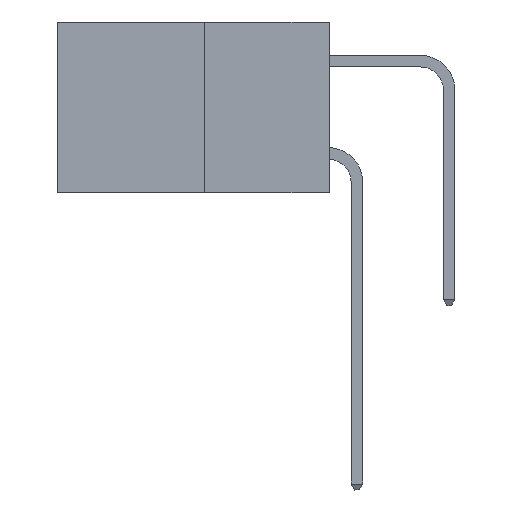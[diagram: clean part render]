
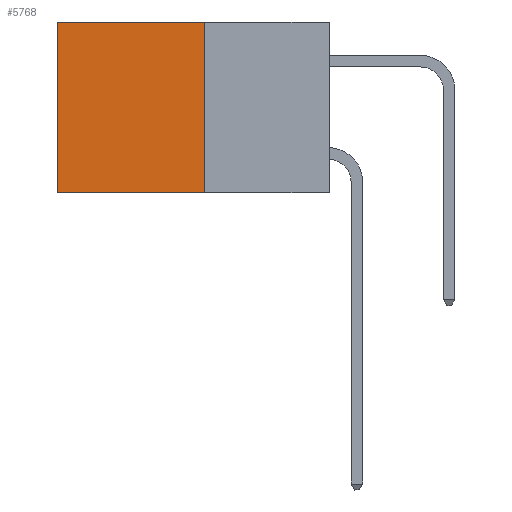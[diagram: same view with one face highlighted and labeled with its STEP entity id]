
A CAD part, left-side view. The second image highlights one B-rep face of the part: STEP entity #5768.
In plain terms, the highlighted planar face has unit normal (-1, 0, 0).
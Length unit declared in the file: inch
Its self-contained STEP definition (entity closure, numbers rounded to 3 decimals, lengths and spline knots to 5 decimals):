
#356 = CARTESIAN_POINT ( 'NONE',  ( 0.277, 0.27, -0.37 ) ) ;
#389 = VERTEX_POINT ( 'NONE', #7781 ) ;
#3956 = CARTESIAN_POINT ( 'NONE',  ( 0.277, 0.27, -0.37 ) ) ;
#4739 = VECTOR ( 'NONE', #16791, 39.37008 ) ;
#4917 = ORIENTED_EDGE ( 'NONE', *, *, #9083, .F. ) ;
#5041 = LINE ( 'NONE', #356, #25148 ) ;
#5121 = PLANE ( 'NONE',  #22793 ) ;
#5768 = ADVANCED_FACE ( 'NONE', ( #12436 ), #5121, .F. ) ;
#5846 = CARTESIAN_POINT ( 'NONE',  ( 0.277, 0.27, 0. ) ) ;
#6281 = DIRECTION ( 'NONE',  ( 0., 0., -1. ) ) ;
#6691 = DIRECTION ( 'NONE',  ( 0., 0., -1. ) ) ;
#7781 = CARTESIAN_POINT ( 'NONE',  ( 0.277, 0.59, -0.37 ) ) ;
#8143 = CARTESIAN_POINT ( 'NONE',  ( 0.277, 0.59, 0. ) ) ;
#9062 = DIRECTION ( 'NONE',  ( 0., 0., -1. ) ) ;
#9083 = EDGE_CURVE ( 'NONE', #11509, #16368, #5041, .T. ) ;
#9275 = EDGE_LOOP ( 'NONE', ( #20755, #25209, #4917, #24793 ) ) ;
#11509 = VERTEX_POINT ( 'NONE', #5846 ) ;
#12280 = DIRECTION ( 'NONE',  ( 0., 1., 0. ) ) ;
#12358 = VECTOR ( 'NONE', #6691, 39.37008 ) ;
#12436 = FACE_OUTER_BOUND ( 'NONE', #9275, .T. ) ;
#14859 = CARTESIAN_POINT ( 'NONE',  ( 0.277, 0.27, -0.37 ) ) ;
#15082 = VERTEX_POINT ( 'NONE', #8143 ) ;
#15148 = LINE ( 'NONE', #14859, #4739 ) ;
#16368 = VERTEX_POINT ( 'NONE', #3956 ) ;
#16402 = CARTESIAN_POINT ( 'NONE',  ( 0.277, 0.59, -0.37 ) ) ;
#16791 = DIRECTION ( 'NONE',  ( 0., 1., 0. ) ) ;
#17236 = EDGE_CURVE ( 'NONE', #11509, #15082, #20643, .T. ) ;
#18718 = CARTESIAN_POINT ( 'NONE',  ( 0.277, 0.27, -0.37 ) ) ;
#20643 = LINE ( 'NONE', #22011, #25210 ) ;
#20702 = DIRECTION ( 'NONE',  ( 1., 0., 0. ) ) ;
#20755 = ORIENTED_EDGE ( 'NONE', *, *, #24052, .T. ) ;
#22011 = CARTESIAN_POINT ( 'NONE',  ( 0.277, 0.27, 0. ) ) ;
#22730 = LINE ( 'NONE', #16402, #12358 ) ;
#22793 = AXIS2_PLACEMENT_3D ( 'NONE', #18718, #20702, #9062 ) ;
#24052 = EDGE_CURVE ( 'NONE', #15082, #389, #22730, .T. ) ;
#24379 = EDGE_CURVE ( 'NONE', #16368, #389, #15148, .T. ) ;
#24793 = ORIENTED_EDGE ( 'NONE', *, *, #17236, .T. ) ;
#25148 = VECTOR ( 'NONE', #6281, 39.37008 ) ;
#25209 = ORIENTED_EDGE ( 'NONE', *, *, #24379, .F. ) ;
#25210 = VECTOR ( 'NONE', #12280, 39.37008 ) ;
